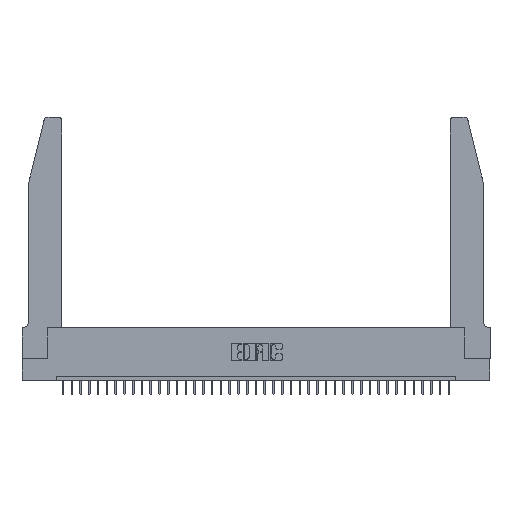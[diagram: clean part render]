
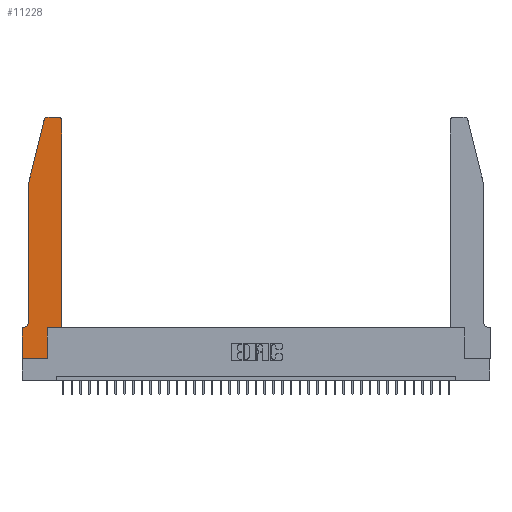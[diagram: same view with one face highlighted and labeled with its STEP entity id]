
A CAD part, top view. The second image highlights one B-rep face of the part: STEP entity #11228.
In plain terms, the highlighted planar face has unit normal (0, 0, 1).
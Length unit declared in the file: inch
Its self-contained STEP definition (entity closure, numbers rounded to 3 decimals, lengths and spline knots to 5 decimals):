
#204 = ORIENTED_EDGE ( 'NONE', *, *, #7134, .T. ) ;
#258 = EDGE_CURVE ( 'NONE', #10905, #5574, #6436, .T. ) ;
#455 = DIRECTION ( 'NONE',  ( -1., 0., 0. ) ) ;
#782 = DIRECTION ( 'NONE',  ( 1., 0., 0. ) ) ;
#866 = VECTOR ( 'NONE', #17783, 39.37008 ) ;
#1490 = EDGE_LOOP ( 'NONE', ( #31735, #34000, #34240, #23229, #24562, #33638, #18609, #33233, #36591, #204, #8350, #24171 ) ) ;
#2364 = VECTOR ( 'NONE', #7992, 39.37008 ) ;
#2673 = AXIS2_PLACEMENT_3D ( 'NONE', #22168, #33634, #31031 ) ;
#3119 = VERTEX_POINT ( 'NONE', #21494 ) ;
#4160 = AXIS2_PLACEMENT_3D ( 'NONE', #28701, #5399, #11028 ) ;
#5399 = DIRECTION ( 'NONE',  ( 0., 0., 1. ) ) ;
#5539 = CARTESIAN_POINT ( 'NONE',  ( 0.0755, 2., 0.37 ) ) ;
#5542 = CIRCLE ( 'NONE', #2673, 0.03 ) ;
#5574 = VERTEX_POINT ( 'NONE', #26634 ) ;
#5590 = VECTOR ( 'NONE', #782, 39.37008 ) ;
#6102 = DIRECTION ( 'NONE',  ( -1., 0., 0. ) ) ;
#6436 = LINE ( 'NONE', #26904, #866 ) ;
#6817 = CARTESIAN_POINT ( 'NONE',  ( 0.284, 2.75, 0.37 ) ) ;
#7134 = EDGE_CURVE ( 'NONE', #9067, #30683, #28089, .T. ) ;
#7992 = DIRECTION ( 'NONE',  ( 0., 1., 0. ) ) ;
#8187 = LINE ( 'NONE', #18037, #9518 ) ;
#8350 = ORIENTED_EDGE ( 'NONE', *, *, #13255, .T. ) ;
#8395 = DIRECTION ( 'NONE',  ( 1., 0., 0. ) ) ;
#8903 = LINE ( 'NONE', #38028, #14071 ) ;
#9053 = LINE ( 'NONE', #12069, #9998 ) ;
#9067 = VERTEX_POINT ( 'NONE', #36915 ) ;
#9518 = VECTOR ( 'NONE', #21105, 39.37008 ) ;
#9781 = LINE ( 'NONE', #34577, #2364 ) ;
#9998 = VECTOR ( 'NONE', #455, 39.37008 ) ;
#10905 = VERTEX_POINT ( 'NONE', #25474 ) ;
#11028 = DIRECTION ( 'NONE',  ( 1., 0., 0. ) ) ;
#11128 = CARTESIAN_POINT ( 'NONE',  ( 0.0755, 0.42, 0.37 ) ) ;
#11228 = ADVANCED_FACE ( 'NONE', ( #15789 ), #25709, .T. ) ;
#11234 = EDGE_CURVE ( 'NONE', #20029, #36395, #35537, .T. ) ;
#11640 = EDGE_CURVE ( 'NONE', #34722, #12111, #22243, .T. ) ;
#11698 = EDGE_CURVE ( 'NONE', #23172, #3119, #5542, .T. ) ;
#12069 = CARTESIAN_POINT ( 'NONE',  ( 0.2605, 2.75, 0.37 ) ) ;
#12111 = VERTEX_POINT ( 'NONE', #19691 ) ;
#12113 = AXIS2_PLACEMENT_3D ( 'NONE', #14143, #37669, #8395 ) ;
#12329 = VECTOR ( 'NONE', #35221, 39.37008 ) ;
#13061 = VECTOR ( 'NONE', #6102, 39.37008 ) ;
#13255 = EDGE_CURVE ( 'NONE', #30683, #23172, #8903, .T. ) ;
#13510 = CARTESIAN_POINT ( 'NONE',  ( 0.0055, 0.42, 0.37 ) ) ;
#13634 = DIRECTION ( 'NONE',  ( -1., 0., 0. ) ) ;
#13836 = CARTESIAN_POINT ( 'NONE',  ( 0.25487, 2.72718, 0.37 ) ) ;
#14071 = VECTOR ( 'NONE', #32595, 39.37008 ) ;
#14143 = CARTESIAN_POINT ( 'NONE',  ( 0.284, 2.72, 0.37 ) ) ;
#14361 = DIRECTION ( 'NONE',  ( 0., -1., 0. ) ) ;
#14432 = CARTESIAN_POINT ( 'NONE',  ( 0.4505, 0.35, 0.37 ) ) ;
#15789 = FACE_OUTER_BOUND ( 'NONE', #1490, .T. ) ;
#15846 = CARTESIAN_POINT ( 'NONE',  ( 0.2865, 0., 0.37 ) ) ;
#17783 = DIRECTION ( 'NONE',  ( 0., -1., 0. ) ) ;
#18037 = CARTESIAN_POINT ( 'NONE',  ( 0.0755, 2., 0.37 ) ) ;
#18609 = ORIENTED_EDGE ( 'NONE', *, *, #258, .T. ) ;
#19691 = CARTESIAN_POINT ( 'NONE',  ( 0.0055, 0.35, 0.37 ) ) ;
#20029 = VERTEX_POINT ( 'NONE', #6817 ) ;
#20069 = AXIS2_PLACEMENT_3D ( 'NONE', #13510, #25351, #13634 ) ;
#20873 = LINE ( 'NONE', #29967, #13061 ) ;
#21105 = DIRECTION ( 'NONE',  ( -0.239, -0.971, 0. ) ) ;
#21494 = CARTESIAN_POINT ( 'NONE',  ( 0.4205, 2.75, 0.37 ) ) ;
#21834 = VERTEX_POINT ( 'NONE', #5539 ) ;
#22065 = VECTOR ( 'NONE', #14361, 39.37008 ) ;
#22168 = CARTESIAN_POINT ( 'NONE',  ( 0.4205, 2.72, 0.37 ) ) ;
#22243 = CIRCLE ( 'NONE', #20069, 0.07 ) ;
#23049 = EDGE_CURVE ( 'NONE', #36395, #21834, #8187, .T. ) ;
#23172 = VERTEX_POINT ( 'NONE', #28273 ) ;
#23229 = ORIENTED_EDGE ( 'NONE', *, *, #38168, .T. ) ;
#24171 = ORIENTED_EDGE ( 'NONE', *, *, #11698, .T. ) ;
#24356 = VERTEX_POINT ( 'NONE', #15846 ) ;
#24538 = LINE ( 'NONE', #30649, #5590 ) ;
#24562 = ORIENTED_EDGE ( 'NONE', *, *, #11640, .T. ) ;
#25208 = EDGE_CURVE ( 'NONE', #3119, #20029, #9053, .T. ) ;
#25351 = DIRECTION ( 'NONE',  ( 0., 0., -1. ) ) ;
#25474 = CARTESIAN_POINT ( 'NONE',  ( 0., 0.35, 0.37 ) ) ;
#25709 = PLANE ( 'NONE',  #4160 ) ;
#26634 = CARTESIAN_POINT ( 'NONE',  ( 0., 0., 0.37 ) ) ;
#26904 = CARTESIAN_POINT ( 'NONE',  ( 0., 0., 0.37 ) ) ;
#28089 = LINE ( 'NONE', #14432, #12329 ) ;
#28255 = EDGE_CURVE ( 'NONE', #24356, #9067, #9781, .T. ) ;
#28273 = CARTESIAN_POINT ( 'NONE',  ( 0.4505, 2.72, 0.37 ) ) ;
#28564 = EDGE_CURVE ( 'NONE', #12111, #10905, #20873, .T. ) ;
#28701 = CARTESIAN_POINT ( 'NONE',  ( 0., 0.35, 0.37 ) ) ;
#29967 = CARTESIAN_POINT ( 'NONE',  ( 0.0755, 0.35, 0.37 ) ) ;
#30289 = LINE ( 'NONE', #31971, #22065 ) ;
#30649 = CARTESIAN_POINT ( 'NONE',  ( 0., 0., 0.37 ) ) ;
#30683 = VERTEX_POINT ( 'NONE', #33460 ) ;
#31031 = DIRECTION ( 'NONE',  ( 1., 0., 0. ) ) ;
#31735 = ORIENTED_EDGE ( 'NONE', *, *, #25208, .T. ) ;
#31805 = EDGE_CURVE ( 'NONE', #5574, #24356, #24538, .T. ) ;
#31971 = CARTESIAN_POINT ( 'NONE',  ( 0.0755, 2., 0.37 ) ) ;
#32595 = DIRECTION ( 'NONE',  ( 0., 1., 0. ) ) ;
#33233 = ORIENTED_EDGE ( 'NONE', *, *, #31805, .T. ) ;
#33460 = CARTESIAN_POINT ( 'NONE',  ( 0.4505, 0.35, 0.37 ) ) ;
#33634 = DIRECTION ( 'NONE',  ( 0., 0., 1. ) ) ;
#33638 = ORIENTED_EDGE ( 'NONE', *, *, #28564, .T. ) ;
#34000 = ORIENTED_EDGE ( 'NONE', *, *, #11234, .T. ) ;
#34240 = ORIENTED_EDGE ( 'NONE', *, *, #23049, .T. ) ;
#34577 = CARTESIAN_POINT ( 'NONE',  ( 0.2865, 0.35, 0.37 ) ) ;
#34722 = VERTEX_POINT ( 'NONE', #11128 ) ;
#35221 = DIRECTION ( 'NONE',  ( 1., 0., 0. ) ) ;
#35537 = CIRCLE ( 'NONE', #12113, 0.03 ) ;
#36395 = VERTEX_POINT ( 'NONE', #13836 ) ;
#36591 = ORIENTED_EDGE ( 'NONE', *, *, #28255, .T. ) ;
#36915 = CARTESIAN_POINT ( 'NONE',  ( 0.2865, 0.35, 0.37 ) ) ;
#37669 = DIRECTION ( 'NONE',  ( 0., 0., 1. ) ) ;
#38028 = CARTESIAN_POINT ( 'NONE',  ( 0.4505, 0.35, 0.37 ) ) ;
#38168 = EDGE_CURVE ( 'NONE', #21834, #34722, #30289, .T. ) ;
